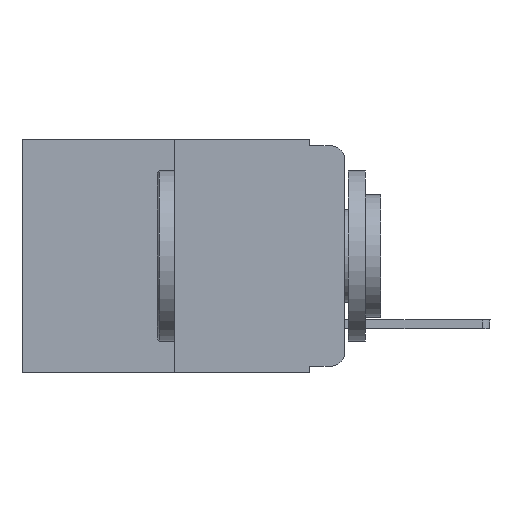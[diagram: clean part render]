
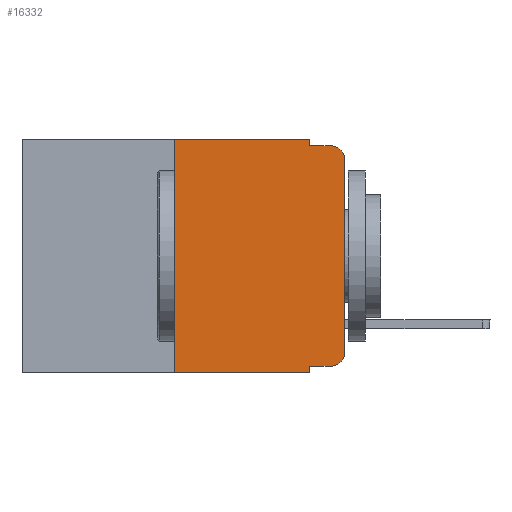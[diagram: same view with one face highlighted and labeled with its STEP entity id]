
A CAD part, left-side view. The second image highlights one B-rep face of the part: STEP entity #16332.
In plain terms, the highlighted planar face has unit normal (-1, 0, 0).
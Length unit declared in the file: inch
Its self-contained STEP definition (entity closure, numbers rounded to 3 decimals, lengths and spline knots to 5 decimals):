
#287 = EDGE_CURVE ( 'NONE', #7948, #3557, #10370, .T. ) ;
#304 = DIRECTION ( 'NONE',  ( 0., 0., -1. ) ) ;
#526 = LINE ( 'NONE', #11083, #18068 ) ;
#893 = EDGE_CURVE ( 'NONE', #8120, #5974, #6918, .T. ) ;
#1014 = FACE_OUTER_BOUND ( 'NONE', #12817, .T. ) ;
#1033 = CARTESIAN_POINT ( 'NONE',  ( 0., 0.02, -0.333 ) ) ;
#1242 = LINE ( 'NONE', #3039, #14386 ) ;
#1944 = CARTESIAN_POINT ( 'NONE',  ( 0., 0.02, -0.313 ) ) ;
#2339 = ORIENTED_EDGE ( 'NONE', *, *, #8400, .F. ) ;
#2753 = CARTESIAN_POINT ( 'NONE',  ( 0., 0.051, -0.343 ) ) ;
#3039 = CARTESIAN_POINT ( 'NONE',  ( 0., 0.25, 0. ) ) ;
#3045 = EDGE_CURVE ( 'NONE', #9648, #16092, #8247, .T. ) ;
#3404 = AXIS2_PLACEMENT_3D ( 'NONE', #18295, #16936, #13821 ) ;
#3492 = DIRECTION ( 'NONE',  ( -1., 0., 0. ) ) ;
#3557 = VERTEX_POINT ( 'NONE', #2753 ) ;
#3819 = CARTESIAN_POINT ( 'NONE',  ( 0., 0.25, -0.343 ) ) ;
#3909 = ORIENTED_EDGE ( 'NONE', *, *, #3045, .T. ) ;
#4264 = LINE ( 'NONE', #8305, #12094 ) ;
#4412 = CARTESIAN_POINT ( 'NONE',  ( 0., 0.473, -0.343 ) ) ;
#4594 = VECTOR ( 'NONE', #12017, 39.37008 ) ;
#4637 = DIRECTION ( 'NONE',  ( 0., 0., -1. ) ) ;
#4972 = ORIENTED_EDGE ( 'NONE', *, *, #20059, .F. ) ;
#5010 = CARTESIAN_POINT ( 'NONE',  ( 0., 0.473, 0. ) ) ;
#5112 = VECTOR ( 'NONE', #6524, 39.37008 ) ;
#5558 = EDGE_CURVE ( 'NONE', #7948, #9648, #4264, .T. ) ;
#5620 = LINE ( 'NONE', #9678, #5112 ) ;
#5630 = VECTOR ( 'NONE', #16140, 39.37008 ) ;
#5974 = VERTEX_POINT ( 'NONE', #11294 ) ;
#5987 = CARTESIAN_POINT ( 'NONE',  ( 0., 0., -0.313 ) ) ;
#6105 = DIRECTION ( 'NONE',  ( 0., 0., 1. ) ) ;
#6375 = ORIENTED_EDGE ( 'NONE', *, *, #5558, .T. ) ;
#6524 = DIRECTION ( 'NONE',  ( 0., -1., 0. ) ) ;
#6733 = DIRECTION ( 'NONE',  ( 0., 0., -1. ) ) ;
#6918 = CIRCLE ( 'NONE', #3404, 0.02 ) ;
#7498 = EDGE_CURVE ( 'NONE', #16092, #8120, #18562, .T. ) ;
#7682 = EDGE_CURVE ( 'NONE', #15944, #3557, #17107, .T. ) ;
#7948 = VERTEX_POINT ( 'NONE', #9872 ) ;
#8120 = VERTEX_POINT ( 'NONE', #11783 ) ;
#8247 = CIRCLE ( 'NONE', #13897, 0.02 ) ;
#8305 = CARTESIAN_POINT ( 'NONE',  ( 0., 0.051, -0.333 ) ) ;
#8400 = EDGE_CURVE ( 'NONE', #15944, #11989, #1242, .T. ) ;
#9054 = CARTESIAN_POINT ( 'NONE',  ( 0., 0.051, -0.01 ) ) ;
#9626 = ORIENTED_EDGE ( 'NONE', *, *, #11143, .F. ) ;
#9627 = CARTESIAN_POINT ( 'NONE',  ( 0., 0.051, 0. ) ) ;
#9648 = VERTEX_POINT ( 'NONE', #1033 ) ;
#9678 = CARTESIAN_POINT ( 'NONE',  ( 0., 0.473, 0. ) ) ;
#9872 = CARTESIAN_POINT ( 'NONE',  ( 0., 0.051, -0.333 ) ) ;
#10112 = VECTOR ( 'NONE', #304, 39.37008 ) ;
#10370 = LINE ( 'NONE', #9627, #10112 ) ;
#10874 = VERTEX_POINT ( 'NONE', #19765 ) ;
#11083 = CARTESIAN_POINT ( 'NONE',  ( 0., 0.051, 0. ) ) ;
#11143 = EDGE_CURVE ( 'NONE', #10874, #16505, #526, .T. ) ;
#11261 = DIRECTION ( 'NONE',  ( 1., 0., 0. ) ) ;
#11294 = CARTESIAN_POINT ( 'NONE',  ( 0., 0.02, -0.01 ) ) ;
#11589 = CARTESIAN_POINT ( 'NONE',  ( 0., 0., 0. ) ) ;
#11673 = DIRECTION ( 'NONE',  ( 0., -1., 0. ) ) ;
#11783 = CARTESIAN_POINT ( 'NONE',  ( 0., 0., -0.03 ) ) ;
#11989 = VERTEX_POINT ( 'NONE', #14822 ) ;
#12017 = DIRECTION ( 'NONE',  ( 0., -1., 0. ) ) ;
#12094 = VECTOR ( 'NONE', #11673, 39.37008 ) ;
#12817 = EDGE_LOOP ( 'NONE', ( #16262, #16468, #4972, #9626, #16329, #2339, #19716, #15937, #6375, #3909 ) ) ;
#12840 = DIRECTION ( 'NONE',  ( 0., 0., -1. ) ) ;
#12978 = VECTOR ( 'NONE', #13361, 39.37008 ) ;
#13088 = CARTESIAN_POINT ( 'NONE',  ( 0., 0.051, -0.01 ) ) ;
#13361 = DIRECTION ( 'NONE',  ( 0., -1., 0. ) ) ;
#13402 = LINE ( 'NONE', #9054, #4594 ) ;
#13821 = DIRECTION ( 'NONE',  ( 0., 0., -1. ) ) ;
#13897 = AXIS2_PLACEMENT_3D ( 'NONE', #1944, #3492, #12840 ) ;
#14386 = VECTOR ( 'NONE', #6105, 39.37008 ) ;
#14822 = CARTESIAN_POINT ( 'NONE',  ( 0., 0.25, 0. ) ) ;
#15560 = AXIS2_PLACEMENT_3D ( 'NONE', #5010, #11261, #6733 ) ;
#15864 = PLANE ( 'NONE',  #15560 ) ;
#15937 = ORIENTED_EDGE ( 'NONE', *, *, #287, .F. ) ;
#15944 = VERTEX_POINT ( 'NONE', #3819 ) ;
#16092 = VERTEX_POINT ( 'NONE', #5987 ) ;
#16140 = DIRECTION ( 'NONE',  ( 0., 0., 1. ) ) ;
#16262 = ORIENTED_EDGE ( 'NONE', *, *, #7498, .T. ) ;
#16298 = EDGE_CURVE ( 'NONE', #11989, #10874, #5620, .T. ) ;
#16329 = ORIENTED_EDGE ( 'NONE', *, *, #16298, .F. ) ;
#16332 = ADVANCED_FACE ( 'NONE', ( #1014 ), #15864, .F. ) ;
#16468 = ORIENTED_EDGE ( 'NONE', *, *, #893, .T. ) ;
#16505 = VERTEX_POINT ( 'NONE', #13088 ) ;
#16936 = DIRECTION ( 'NONE',  ( -1., 0., 0. ) ) ;
#17107 = LINE ( 'NONE', #4412, #12978 ) ;
#18068 = VECTOR ( 'NONE', #4637, 39.37008 ) ;
#18295 = CARTESIAN_POINT ( 'NONE',  ( 0., 0.02, -0.03 ) ) ;
#18562 = LINE ( 'NONE', #11589, #5630 ) ;
#19716 = ORIENTED_EDGE ( 'NONE', *, *, #7682, .T. ) ;
#19765 = CARTESIAN_POINT ( 'NONE',  ( 0., 0.051, 0. ) ) ;
#20059 = EDGE_CURVE ( 'NONE', #16505, #5974, #13402, .T. ) ;
